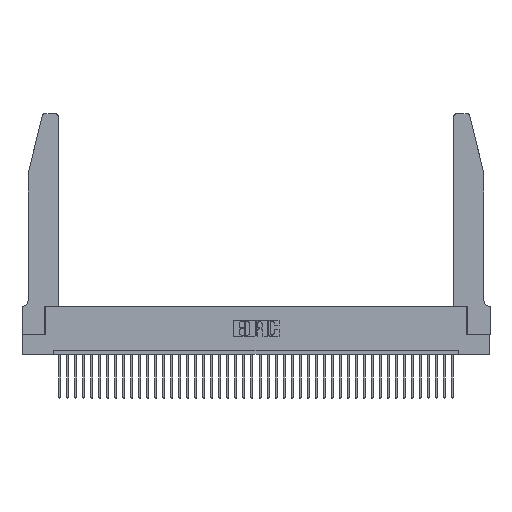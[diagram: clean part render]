
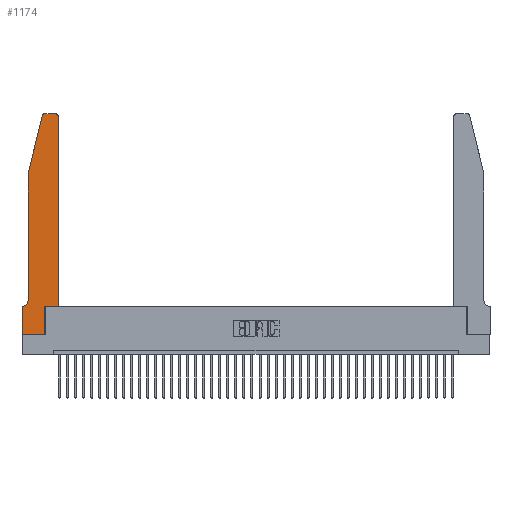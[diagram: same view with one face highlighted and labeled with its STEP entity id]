
A CAD part, top view. The second image highlights one B-rep face of the part: STEP entity #1174.
In plain terms, the highlighted planar face has unit normal (0, 0, 1).
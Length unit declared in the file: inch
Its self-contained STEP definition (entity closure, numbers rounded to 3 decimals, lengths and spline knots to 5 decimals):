
#787 = ORIENTED_EDGE ( 'NONE', *, *, #25380, .T. ) ;
#974 = CARTESIAN_POINT ( 'NONE',  ( 0.0755, 2., 0.37 ) ) ;
#1174 = ADVANCED_FACE ( 'NONE', ( #14834 ), #20985, .T. ) ;
#1464 = EDGE_CURVE ( 'NONE', #8635, #4522, #31759, .T. ) ;
#1610 = ORIENTED_EDGE ( 'NONE', *, *, #39066, .T. ) ;
#2237 = VECTOR ( 'NONE', #38261, 39.37008 ) ;
#2832 = VERTEX_POINT ( 'NONE', #22820 ) ;
#3624 = LINE ( 'NONE', #25196, #2237 ) ;
#3655 = VECTOR ( 'NONE', #23196, 39.37008 ) ;
#3976 = EDGE_CURVE ( 'NONE', #20257, #35887, #19194, .T. ) ;
#4299 = CARTESIAN_POINT ( 'NONE',  ( 0., 0., 0.37 ) ) ;
#4522 = VERTEX_POINT ( 'NONE', #33209 ) ;
#4576 = DIRECTION ( 'NONE',  ( 1., 0., 0. ) ) ;
#4891 = DIRECTION ( 'NONE',  ( 0., -1., 0. ) ) ;
#5272 = DIRECTION ( 'NONE',  ( -1., 0., 0. ) ) ;
#5804 = ORIENTED_EDGE ( 'NONE', *, *, #6730, .T. ) ;
#5995 = VERTEX_POINT ( 'NONE', #11926 ) ;
#6709 = VERTEX_POINT ( 'NONE', #36946 ) ;
#6730 = EDGE_CURVE ( 'NONE', #4522, #11592, #6904, .T. ) ;
#6904 = LINE ( 'NONE', #14691, #38848 ) ;
#7484 = EDGE_CURVE ( 'NONE', #31042, #20257, #10414, .T. ) ;
#7880 = CARTESIAN_POINT ( 'NONE',  ( 0.0055, 0.42, 0.37 ) ) ;
#8635 = VERTEX_POINT ( 'NONE', #31037 ) ;
#8739 = LINE ( 'NONE', #20741, #11230 ) ;
#9238 = VECTOR ( 'NONE', #24726, 39.37008 ) ;
#10414 = CIRCLE ( 'NONE', #11958, 0.07 ) ;
#11230 = VECTOR ( 'NONE', #14468, 39.37008 ) ;
#11592 = VERTEX_POINT ( 'NONE', #37465 ) ;
#11926 = CARTESIAN_POINT ( 'NONE',  ( 0.2865, 0.35, 0.37 ) ) ;
#11958 = AXIS2_PLACEMENT_3D ( 'NONE', #7880, #29599, #5272 ) ;
#12000 = CARTESIAN_POINT ( 'NONE',  ( 0.0755, 0.42, 0.37 ) ) ;
#13210 = VECTOR ( 'NONE', #19984, 39.37008 ) ;
#13438 = ORIENTED_EDGE ( 'NONE', *, *, #32138, .T. ) ;
#13710 = CIRCLE ( 'NONE', #35862, 0.03 ) ;
#14062 = ORIENTED_EDGE ( 'NONE', *, *, #7484, .T. ) ;
#14171 = VERTEX_POINT ( 'NONE', #40256 ) ;
#14468 = DIRECTION ( 'NONE',  ( -1., 0., 0. ) ) ;
#14691 = CARTESIAN_POINT ( 'NONE',  ( 0.0755, 2., 0.37 ) ) ;
#14834 = FACE_OUTER_BOUND ( 'NONE', #40435, .T. ) ;
#15067 = DIRECTION ( 'NONE',  ( 0., 1., 0. ) ) ;
#17078 = LINE ( 'NONE', #4299, #39017 ) ;
#18330 = DIRECTION ( 'NONE',  ( 0., 1., 0. ) ) ;
#18780 = VECTOR ( 'NONE', #18330, 39.37008 ) ;
#19065 = EDGE_CURVE ( 'NONE', #30027, #26308, #3624, .T. ) ;
#19194 = LINE ( 'NONE', #27889, #9238 ) ;
#19222 = LINE ( 'NONE', #34590, #18780 ) ;
#19984 = DIRECTION ( 'NONE',  ( 1., 0., 0. ) ) ;
#20257 = VERTEX_POINT ( 'NONE', #25201 ) ;
#20741 = CARTESIAN_POINT ( 'NONE',  ( 0.2605, 2.75, 0.37 ) ) ;
#20985 = PLANE ( 'NONE',  #35173 ) ;
#21180 = ORIENTED_EDGE ( 'NONE', *, *, #3976, .T. ) ;
#21507 = ORIENTED_EDGE ( 'NONE', *, *, #39212, .T. ) ;
#22045 = ORIENTED_EDGE ( 'NONE', *, *, #1464, .T. ) ;
#22820 = CARTESIAN_POINT ( 'NONE',  ( 0.4205, 2.75, 0.37 ) ) ;
#23196 = DIRECTION ( 'NONE',  ( 0., -1., 0. ) ) ;
#23407 = LINE ( 'NONE', #33692, #23962 ) ;
#23737 = AXIS2_PLACEMENT_3D ( 'NONE', #38787, #29002, #31951 ) ;
#23880 = DIRECTION ( 'NONE',  ( 1., 0., 0. ) ) ;
#23962 = VECTOR ( 'NONE', #15067, 39.37008 ) ;
#24025 = CARTESIAN_POINT ( 'NONE',  ( 0.4205, 2.72, 0.37 ) ) ;
#24171 = DIRECTION ( 'NONE',  ( 0., 0., 1. ) ) ;
#24179 = DIRECTION ( 'NONE',  ( 0., 0., 1. ) ) ;
#24726 = DIRECTION ( 'NONE',  ( -1., 0., 0. ) ) ;
#25084 = EDGE_CURVE ( 'NONE', #5995, #6709, #31697, .T. ) ;
#25196 = CARTESIAN_POINT ( 'NONE',  ( 0., 0., 0.37 ) ) ;
#25201 = CARTESIAN_POINT ( 'NONE',  ( 0.0055, 0.35, 0.37 ) ) ;
#25316 = CARTESIAN_POINT ( 'NONE',  ( 0., 0.35, 0.37 ) ) ;
#25380 = EDGE_CURVE ( 'NONE', #6709, #14171, #19222, .T. ) ;
#25863 = EDGE_CURVE ( 'NONE', #14171, #2832, #13710, .T. ) ;
#25976 = ORIENTED_EDGE ( 'NONE', *, *, #36245, .T. ) ;
#26308 = VERTEX_POINT ( 'NONE', #32542 ) ;
#26801 = CARTESIAN_POINT ( 'NONE',  ( 0.4505, 0.35, 0.37 ) ) ;
#27889 = CARTESIAN_POINT ( 'NONE',  ( 0.0755, 0.35, 0.37 ) ) ;
#28175 = LINE ( 'NONE', #974, #3655 ) ;
#29002 = DIRECTION ( 'NONE',  ( 0., 0., 1. ) ) ;
#29599 = DIRECTION ( 'NONE',  ( 0., 0., -1. ) ) ;
#30027 = VERTEX_POINT ( 'NONE', #36116 ) ;
#30523 = DIRECTION ( 'NONE',  ( -0.239, -0.971, 0. ) ) ;
#30671 = ORIENTED_EDGE ( 'NONE', *, *, #25863, .T. ) ;
#30691 = CARTESIAN_POINT ( 'NONE',  ( 0., 0.35, 0.37 ) ) ;
#31037 = CARTESIAN_POINT ( 'NONE',  ( 0.284, 2.75, 0.37 ) ) ;
#31042 = VERTEX_POINT ( 'NONE', #12000 ) ;
#31697 = LINE ( 'NONE', #26801, #13210 ) ;
#31759 = CIRCLE ( 'NONE', #23737, 0.03 ) ;
#31951 = DIRECTION ( 'NONE',  ( 1., 0., 0. ) ) ;
#32138 = EDGE_CURVE ( 'NONE', #26308, #5995, #23407, .T. ) ;
#32542 = CARTESIAN_POINT ( 'NONE',  ( 0.2865, 0., 0.37 ) ) ;
#32643 = ORIENTED_EDGE ( 'NONE', *, *, #19065, .T. ) ;
#33209 = CARTESIAN_POINT ( 'NONE',  ( 0.25487, 2.72718, 0.37 ) ) ;
#33692 = CARTESIAN_POINT ( 'NONE',  ( 0.2865, 0.35, 0.37 ) ) ;
#34590 = CARTESIAN_POINT ( 'NONE',  ( 0.4505, 0.35, 0.37 ) ) ;
#35173 = AXIS2_PLACEMENT_3D ( 'NONE', #30691, #24179, #23880 ) ;
#35862 = AXIS2_PLACEMENT_3D ( 'NONE', #24025, #24171, #4576 ) ;
#35887 = VERTEX_POINT ( 'NONE', #25316 ) ;
#36116 = CARTESIAN_POINT ( 'NONE',  ( 0., 0., 0.37 ) ) ;
#36245 = EDGE_CURVE ( 'NONE', #35887, #30027, #17078, .T. ) ;
#36946 = CARTESIAN_POINT ( 'NONE',  ( 0.4505, 0.35, 0.37 ) ) ;
#37465 = CARTESIAN_POINT ( 'NONE',  ( 0.0755, 2., 0.37 ) ) ;
#38261 = DIRECTION ( 'NONE',  ( 1., 0., 0. ) ) ;
#38787 = CARTESIAN_POINT ( 'NONE',  ( 0.284, 2.72, 0.37 ) ) ;
#38848 = VECTOR ( 'NONE', #30523, 39.37008 ) ;
#39017 = VECTOR ( 'NONE', #4891, 39.37008 ) ;
#39066 = EDGE_CURVE ( 'NONE', #11592, #31042, #28175, .T. ) ;
#39212 = EDGE_CURVE ( 'NONE', #2832, #8635, #8739, .T. ) ;
#40256 = CARTESIAN_POINT ( 'NONE',  ( 0.4505, 2.72, 0.37 ) ) ;
#40435 = EDGE_LOOP ( 'NONE', ( #21507, #22045, #5804, #1610, #14062, #21180, #25976, #32643, #13438, #41154, #787, #30671 ) ) ;
#41154 = ORIENTED_EDGE ( 'NONE', *, *, #25084, .T. ) ;
